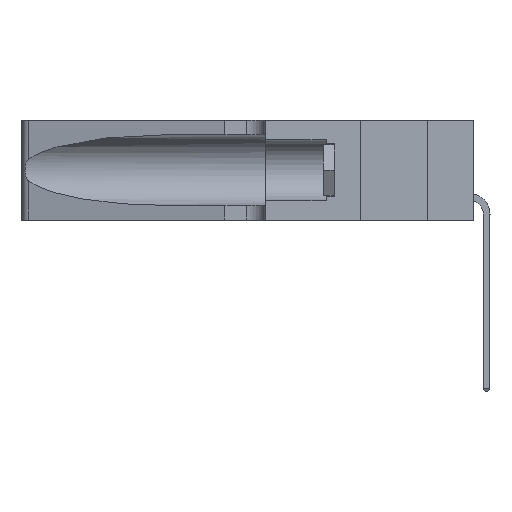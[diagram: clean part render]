
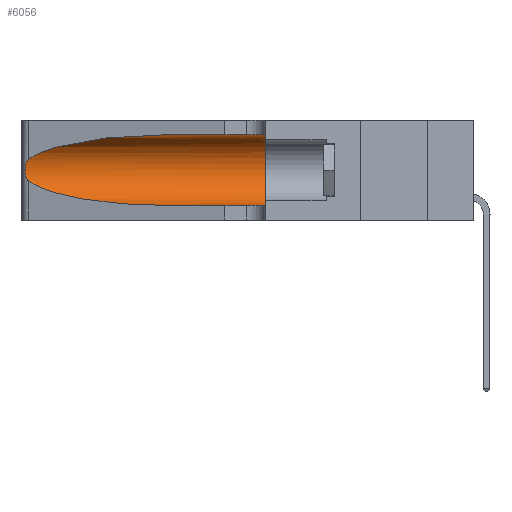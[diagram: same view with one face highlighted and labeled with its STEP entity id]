
A CAD part, left-side view. The second image highlights one B-rep face of the part: STEP entity #6056.
In plain terms, the highlighted cylindrical face has radius 3.308 mm (diameter 6.617 mm), a partial arc.
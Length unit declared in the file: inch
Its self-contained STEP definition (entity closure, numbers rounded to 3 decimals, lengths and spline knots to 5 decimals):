
#918 = CARTESIAN_POINT ( 'NONE',  ( 0.25555, 1.22993, 0.14849 ) ) ;
#2650 =( BOUNDED_CURVE ( )  B_SPLINE_CURVE ( 3, ( #31789, #20966, #7142, #32512 ),
 .UNSPECIFIED., .F., .F. ) 
 B_SPLINE_CURVE_WITH_KNOTS ( ( 4, 4 ),
 ( 3.44316, 4.71239 ),
 .UNSPECIFIED. ) 
 CURVE ( )  GEOMETRIC_REPRESENTATION_ITEM ( )  RATIONAL_B_SPLINE_CURVE ( ( 1., 0.87, 0.87, 1. ) ) 
 REPRESENTATION_ITEM ( '' )  );
#2720 = VERTEX_POINT ( 'NONE', #33502 ) ;
#3433 = EDGE_CURVE ( 'NONE', #10177, #28364, #34679, .T. ) ;
#3591 = CARTESIAN_POINT ( 'NONE',  ( 0.26075, 1.23896, 0.19203 ) ) ;
#3667 = CARTESIAN_POINT ( 'NONE',  ( 0.1305, 0.35, 0.05475 ) ) ;
#6056 = ADVANCED_FACE ( 'NONE', ( #19007 ), #17709, .F. ) ;
#6451 = CARTESIAN_POINT ( 'NONE',  ( 0.1305, 1.61858, 0.31525 ) ) ;
#7142 = CARTESIAN_POINT ( 'NONE',  ( 0.18966, 0.96281, 0.05475 ) ) ;
#7442 = CARTESIAN_POINT ( 'NONE',  ( 0.1305, 0.72297, 0.31525 ) ) ;
#8818 = ORIENTED_EDGE ( 'NONE', *, *, #3433, .F. ) ;
#9012 = CARTESIAN_POINT ( 'NONE',  ( 0.25487, 1.22718, 0.22369 ) ) ;
#9501 = AXIS2_PLACEMENT_3D ( 'NONE', #33459, #33579, #11059 ) ;
#10177 = VERTEX_POINT ( 'NONE', #12130 ) ;
#10759 = CARTESIAN_POINT ( 'NONE',  ( 0.25487, 1.22718, 0.14631 ) ) ;
#10885 = ORIENTED_EDGE ( 'NONE', *, *, #15975, .T. ) ;
#11059 = DIRECTION ( 'NONE',  ( 0., 0., 1. ) ) ;
#11270 = B_SPLINE_CURVE_WITH_KNOTS ( 'NONE', 3,
 ( #34518, #31554, #17632, #31924, #14671, #12095, #3591, #17880, #23332, #28974, #31801, #34642, #918, #20599 ),
 .UNSPECIFIED., .F., .F.,
 ( 4, 2, 2, 2, 2, 2, 4 ),
 ( 0., 0.00027, 0.00053, 0.00107, 0.0016, 0.00187, 0.00214 ),
 .UNSPECIFIED. ) ;
#12055 = VERTEX_POINT ( 'NONE', #12164 ) ;
#12095 = CARTESIAN_POINT ( 'NONE',  ( 0.26018, 1.23835, 0.19895 ) ) ;
#12130 = CARTESIAN_POINT ( 'NONE',  ( 0.1305, 0.35, 0.31525 ) ) ;
#12164 = CARTESIAN_POINT ( 'NONE',  ( 0.25487, 1.22718, 0.22369 ) ) ;
#13271 = EDGE_CURVE ( 'NONE', #12055, #25630, #11270, .T. ) ;
#13381 = AXIS2_PLACEMENT_3D ( 'NONE', #18255, #14935, #15055 ) ;
#14671 = CARTESIAN_POINT ( 'NONE',  ( 0.25854, 1.2359, 0.20912 ) ) ;
#14935 = DIRECTION ( 'NONE',  ( 0., -1., 0. ) ) ;
#15055 = DIRECTION ( 'NONE',  ( 0., 0., -1. ) ) ;
#15975 = EDGE_CURVE ( 'NONE', #17865, #12055, #16170, .T. ) ;
#16170 =( BOUNDED_CURVE ( )  B_SPLINE_CURVE ( 3, ( #26150, #28584, #17361, #9012 ),
 .UNSPECIFIED., .F., .F. ) 
 B_SPLINE_CURVE_WITH_KNOTS ( ( 4, 4 ),
 ( 1.5708, 2.84003 ),
 .UNSPECIFIED. ) 
 CURVE ( )  GEOMETRIC_REPRESENTATION_ITEM ( )  RATIONAL_B_SPLINE_CURVE ( ( 1., 0.87, 0.87, 1. ) ) 
 REPRESENTATION_ITEM ( '' )  );
#17068 = VECTOR ( 'NONE', #28805, 39.37008 ) ;
#17361 = CARTESIAN_POINT ( 'NONE',  ( 0.2373, 1.15595, 0.28018 ) ) ;
#17632 = CARTESIAN_POINT ( 'NONE',  ( 0.25639, 1.23184, 0.21858 ) ) ;
#17709 = CYLINDRICAL_SURFACE ( 'NONE', #13381, 0.13025 ) ;
#17865 = VERTEX_POINT ( 'NONE', #7442 ) ;
#17880 = CARTESIAN_POINT ( 'NONE',  ( 0.26075, 1.23896, 0.178 ) ) ;
#18127 = ORIENTED_EDGE ( 'NONE', *, *, #36432, .T. ) ;
#18255 = CARTESIAN_POINT ( 'NONE',  ( 0.1305, 1.61858, 0.185 ) ) ;
#19007 = FACE_OUTER_BOUND ( 'NONE', #32838, .T. ) ;
#20213 = VECTOR ( 'NONE', #28625, 39.37008 ) ;
#20599 = CARTESIAN_POINT ( 'NONE',  ( 0.25487, 1.22718, 0.14631 ) ) ;
#20966 = CARTESIAN_POINT ( 'NONE',  ( 0.2373, 1.15595, 0.08982 ) ) ;
#21334 = EDGE_CURVE ( 'NONE', #17865, #10177, #28163, .T. ) ;
#21370 = ORIENTED_EDGE ( 'NONE', *, *, #28312, .T. ) ;
#23302 = LINE ( 'NONE', #26126, #17068 ) ;
#23332 = CARTESIAN_POINT ( 'NONE',  ( 0.26017, 1.23833, 0.17102 ) ) ;
#25630 = VERTEX_POINT ( 'NONE', #10759 ) ;
#26126 = CARTESIAN_POINT ( 'NONE',  ( 0.1305, 1.61858, 0.05475 ) ) ;
#26150 = CARTESIAN_POINT ( 'NONE',  ( 0.1305, 0.72297, 0.31525 ) ) ;
#27466 = ORIENTED_EDGE ( 'NONE', *, *, #21334, .F. ) ;
#28163 = LINE ( 'NONE', #6451, #20213 ) ;
#28312 = EDGE_CURVE ( 'NONE', #2720, #28364, #23302, .T. ) ;
#28364 = VERTEX_POINT ( 'NONE', #3667 ) ;
#28584 = CARTESIAN_POINT ( 'NONE',  ( 0.18966, 0.96281, 0.31525 ) ) ;
#28625 = DIRECTION ( 'NONE',  ( 0., -1., 0. ) ) ;
#28805 = DIRECTION ( 'NONE',  ( 0., -1., 0. ) ) ;
#28974 = CARTESIAN_POINT ( 'NONE',  ( 0.25856, 1.23593, 0.16098 ) ) ;
#31554 = CARTESIAN_POINT ( 'NONE',  ( 0.25555, 1.22994, 0.2215 ) ) ;
#31789 = CARTESIAN_POINT ( 'NONE',  ( 0.25487, 1.22718, 0.14631 ) ) ;
#31801 = CARTESIAN_POINT ( 'NONE',  ( 0.25789, 1.23486, 0.15765 ) ) ;
#31924 = CARTESIAN_POINT ( 'NONE',  ( 0.25787, 1.23484, 0.2124 ) ) ;
#32273 = ORIENTED_EDGE ( 'NONE', *, *, #13271, .T. ) ;
#32512 = CARTESIAN_POINT ( 'NONE',  ( 0.1305, 0.72297, 0.05475 ) ) ;
#32838 = EDGE_LOOP ( 'NONE', ( #10885, #32273, #18127, #21370, #8818, #27466 ) ) ;
#33459 = CARTESIAN_POINT ( 'NONE',  ( 0.1305, 0.35, 0.185 ) ) ;
#33502 = CARTESIAN_POINT ( 'NONE',  ( 0.1305, 0.72297, 0.05475 ) ) ;
#33579 = DIRECTION ( 'NONE',  ( 0., 1., 0. ) ) ;
#34518 = CARTESIAN_POINT ( 'NONE',  ( 0.25487, 1.22718, 0.22369 ) ) ;
#34642 = CARTESIAN_POINT ( 'NONE',  ( 0.25639, 1.23186, 0.15144 ) ) ;
#34679 = CIRCLE ( 'NONE', #9501, 0.13025 ) ;
#36432 = EDGE_CURVE ( 'NONE', #25630, #2720, #2650, .T. ) ;
